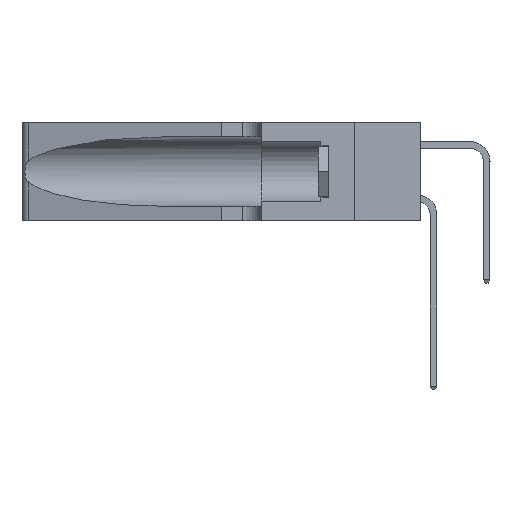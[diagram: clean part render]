
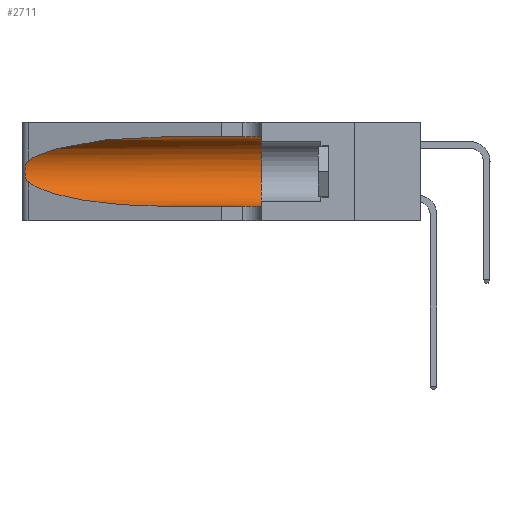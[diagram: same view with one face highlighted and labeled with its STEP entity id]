
A CAD part, left-side view. The second image highlights one B-rep face of the part: STEP entity #2711.
In plain terms, the highlighted cylindrical face has radius 3.308 mm (diameter 6.617 mm), a partial arc.
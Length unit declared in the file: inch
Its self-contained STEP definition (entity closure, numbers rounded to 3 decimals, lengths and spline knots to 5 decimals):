
#25 = CYLINDRICAL_SURFACE ( 'NONE', #16370, 0.13025 ) ;
#465 = DIRECTION ( 'NONE',  ( 0., -1., 0. ) ) ;
#698 = ORIENTED_EDGE ( 'NONE', *, *, #10472, .T. ) ;
#732 = FACE_OUTER_BOUND ( 'NONE', #2163, .T. ) ;
#1047 = CARTESIAN_POINT ( 'NONE',  ( 0.18966, 0.96281, 0.31525 ) ) ;
#1628 = AXIS2_PLACEMENT_3D ( 'NONE', #17911, #5132, #20025 ) ;
#1874 = DIRECTION ( 'NONE',  ( 0., -1., 0. ) ) ;
#2163 = EDGE_LOOP ( 'NONE', ( #698, #3542, #5870, #14657, #25169, #18265 ) ) ;
#2185 = CARTESIAN_POINT ( 'NONE',  ( 0.25789, 1.23486, 0.15765 ) ) ;
#2711 = ADVANCED_FACE ( 'NONE', ( #732 ), #25, .F. ) ;
#3235 = VERTEX_POINT ( 'NONE', #20222 ) ;
#3248 = CIRCLE ( 'NONE', #1628, 0.13025 ) ;
#3286 = CARTESIAN_POINT ( 'NONE',  ( 0.1305, 0.72297, 0.31525 ) ) ;
#3542 = ORIENTED_EDGE ( 'NONE', *, *, #22637, .T. ) ;
#4439 = CARTESIAN_POINT ( 'NONE',  ( 0.25555, 1.22993, 0.14849 ) ) ;
#5109 = VERTEX_POINT ( 'NONE', #13305 ) ;
#5132 = DIRECTION ( 'NONE',  ( 0., 1., 0. ) ) ;
#5513 = CARTESIAN_POINT ( 'NONE',  ( 0.1305, 1.61858, 0.185 ) ) ;
#5529 = CARTESIAN_POINT ( 'NONE',  ( 0.2373, 1.15595, 0.28018 ) ) ;
#5577 = DIRECTION ( 'NONE',  ( 0., 0., -1. ) ) ;
#5661 = B_SPLINE_CURVE_WITH_KNOTS ( 'NONE', 3,
 ( #6563, #19289, #21396, #8758, #23496, #10919, #25594, #13002, #25684, #15139, #2185, #17251, #4439, #19382 ),
 .UNSPECIFIED., .F., .F.,
 ( 4, 2, 2, 2, 2, 2, 4 ),
 ( 0., 0.00027, 0.00053, 0.00107, 0.0016, 0.00187, 0.00214 ),
 .UNSPECIFIED. ) ;
#5804 = EDGE_CURVE ( 'NONE', #3235, #26567, #11569, .T. ) ;
#5870 = ORIENTED_EDGE ( 'NONE', *, *, #10309, .T. ) ;
#6563 = CARTESIAN_POINT ( 'NONE',  ( 0.25487, 1.22718, 0.22369 ) ) ;
#7204 = CARTESIAN_POINT ( 'NONE',  ( 0.1305, 0.35, 0.31525 ) ) ;
#8684 = CARTESIAN_POINT ( 'NONE',  ( 0.1305, 0.35, 0.05475 ) ) ;
#8758 = CARTESIAN_POINT ( 'NONE',  ( 0.25787, 1.23484, 0.2124 ) ) ;
#10309 = EDGE_CURVE ( 'NONE', #24865, #3235, #22484, .T. ) ;
#10472 = EDGE_CURVE ( 'NONE', #5109, #11797, #12709, .T. ) ;
#10919 = CARTESIAN_POINT ( 'NONE',  ( 0.26018, 1.23835, 0.19895 ) ) ;
#11390 = CARTESIAN_POINT ( 'NONE',  ( 0.18966, 0.96281, 0.05475 ) ) ;
#11569 = LINE ( 'NONE', #19549, #27661 ) ;
#11797 = VERTEX_POINT ( 'NONE', #26637 ) ;
#12709 =( BOUNDED_CURVE ( )  B_SPLINE_CURVE ( 3, ( #3286, #1047, #5529, #20398 ),
 .UNSPECIFIED., .F., .F. ) 
 B_SPLINE_CURVE_WITH_KNOTS ( ( 4, 4 ),
 ( 1.5708, 2.84003 ),
 .UNSPECIFIED. ) 
 CURVE ( )  GEOMETRIC_REPRESENTATION_ITEM ( )  RATIONAL_B_SPLINE_CURVE ( ( 1., 0.87, 0.87, 1. ) ) 
 REPRESENTATION_ITEM ( '' )  );
#13002 = CARTESIAN_POINT ( 'NONE',  ( 0.26075, 1.23896, 0.178 ) ) ;
#13305 = CARTESIAN_POINT ( 'NONE',  ( 0.1305, 0.72297, 0.31525 ) ) ;
#14657 = ORIENTED_EDGE ( 'NONE', *, *, #5804, .T. ) ;
#15139 = CARTESIAN_POINT ( 'NONE',  ( 0.25856, 1.23593, 0.16098 ) ) ;
#16370 = AXIS2_PLACEMENT_3D ( 'NONE', #5513, #465, #5577 ) ;
#17251 = CARTESIAN_POINT ( 'NONE',  ( 0.25639, 1.23186, 0.15144 ) ) ;
#17911 = CARTESIAN_POINT ( 'NONE',  ( 0.1305, 0.35, 0.185 ) ) ;
#18265 = ORIENTED_EDGE ( 'NONE', *, *, #23203, .F. ) ;
#19289 = CARTESIAN_POINT ( 'NONE',  ( 0.25555, 1.22994, 0.2215 ) ) ;
#19382 = CARTESIAN_POINT ( 'NONE',  ( 0.25487, 1.22718, 0.14631 ) ) ;
#19549 = CARTESIAN_POINT ( 'NONE',  ( 0.1305, 1.61858, 0.05475 ) ) ;
#19755 = CARTESIAN_POINT ( 'NONE',  ( 0.25487, 1.22718, 0.14631 ) ) ;
#20025 = DIRECTION ( 'NONE',  ( 0., 0., 1. ) ) ;
#20222 = CARTESIAN_POINT ( 'NONE',  ( 0.1305, 0.72297, 0.05475 ) ) ;
#20398 = CARTESIAN_POINT ( 'NONE',  ( 0.25487, 1.22718, 0.22369 ) ) ;
#21396 = CARTESIAN_POINT ( 'NONE',  ( 0.25639, 1.23184, 0.21858 ) ) ;
#21882 = VECTOR ( 'NONE', #1874, 39.37008 ) ;
#22203 = EDGE_CURVE ( 'NONE', #24962, #26567, #3248, .T. ) ;
#22484 =( BOUNDED_CURVE ( )  B_SPLINE_CURVE ( 3, ( #19755, #23891, #11390, #26070 ),
 .UNSPECIFIED., .F., .F. ) 
 B_SPLINE_CURVE_WITH_KNOTS ( ( 4, 4 ),
 ( 3.44316, 4.71239 ),
 .UNSPECIFIED. ) 
 CURVE ( )  GEOMETRIC_REPRESENTATION_ITEM ( )  RATIONAL_B_SPLINE_CURVE ( ( 1., 0.87, 0.87, 1. ) ) 
 REPRESENTATION_ITEM ( '' )  );
#22637 = EDGE_CURVE ( 'NONE', #11797, #24865, #5661, .T. ) ;
#23203 = EDGE_CURVE ( 'NONE', #5109, #24962, #27461, .T. ) ;
#23496 = CARTESIAN_POINT ( 'NONE',  ( 0.25854, 1.2359, 0.20912 ) ) ;
#23765 = CARTESIAN_POINT ( 'NONE',  ( 0.25487, 1.22718, 0.14631 ) ) ;
#23891 = CARTESIAN_POINT ( 'NONE',  ( 0.2373, 1.15595, 0.08982 ) ) ;
#24865 = VERTEX_POINT ( 'NONE', #23765 ) ;
#24962 = VERTEX_POINT ( 'NONE', #7204 ) ;
#25169 = ORIENTED_EDGE ( 'NONE', *, *, #22203, .F. ) ;
#25309 = CARTESIAN_POINT ( 'NONE',  ( 0.1305, 1.61858, 0.31525 ) ) ;
#25594 = CARTESIAN_POINT ( 'NONE',  ( 0.26075, 1.23896, 0.19203 ) ) ;
#25684 = CARTESIAN_POINT ( 'NONE',  ( 0.26017, 1.23833, 0.17102 ) ) ;
#25857 = DIRECTION ( 'NONE',  ( 0., -1., 0. ) ) ;
#26070 = CARTESIAN_POINT ( 'NONE',  ( 0.1305, 0.72297, 0.05475 ) ) ;
#26567 = VERTEX_POINT ( 'NONE', #8684 ) ;
#26637 = CARTESIAN_POINT ( 'NONE',  ( 0.25487, 1.22718, 0.22369 ) ) ;
#27461 = LINE ( 'NONE', #25309, #21882 ) ;
#27661 = VECTOR ( 'NONE', #25857, 39.37008 ) ;
